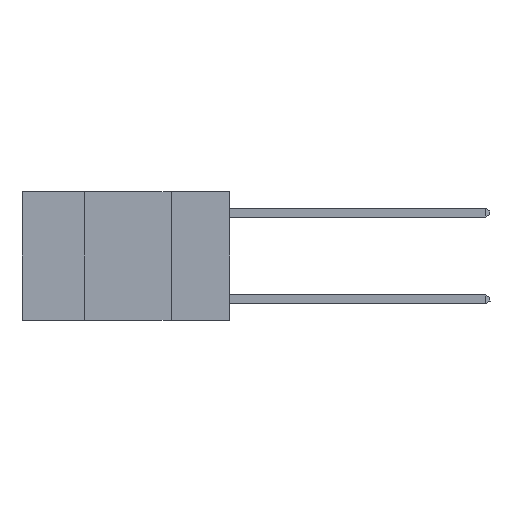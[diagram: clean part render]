
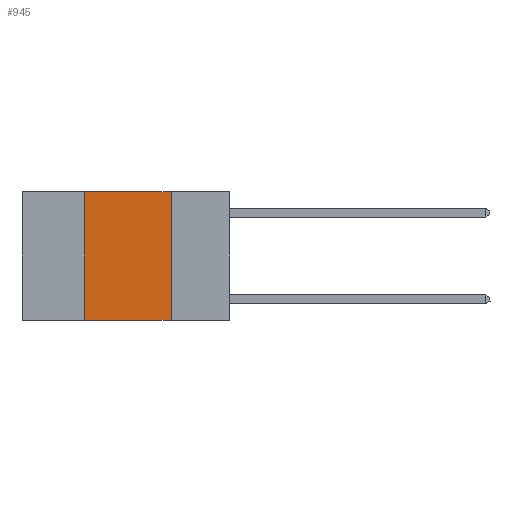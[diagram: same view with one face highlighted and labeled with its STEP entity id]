
A CAD part, left-side view. The second image highlights one B-rep face of the part: STEP entity #945.
In plain terms, the highlighted planar face has unit normal (-1, 0, 0).
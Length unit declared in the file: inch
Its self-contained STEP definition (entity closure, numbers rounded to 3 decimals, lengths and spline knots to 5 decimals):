
#25 = VECTOR ( 'NONE', #1550, 39.37008 ) ;
#100 = EDGE_CURVE ( 'NONE', #499, #8716, #5270, .T. ) ;
#407 = DIRECTION ( 'NONE',  ( 0., -1., 0. ) ) ;
#499 = VERTEX_POINT ( 'NONE', #9473 ) ;
#731 = CARTESIAN_POINT ( 'NONE',  ( 0., 0.17, 0. ) ) ;
#945 = ADVANCED_FACE ( 'NONE', ( #7794 ), #3126, .F. ) ;
#1162 = EDGE_CURVE ( 'NONE', #499, #2624, #2180, .T. ) ;
#1550 = DIRECTION ( 'NONE',  ( 0., 0., -1. ) ) ;
#1669 = VECTOR ( 'NONE', #8028, 39.37008 ) ;
#2180 = LINE ( 'NONE', #4954, #1669 ) ;
#2624 = VERTEX_POINT ( 'NONE', #5604 ) ;
#2625 = LINE ( 'NONE', #9827, #6765 ) ;
#2983 = CARTESIAN_POINT ( 'NONE',  ( 0., 0.17, -0.37 ) ) ;
#3094 = VERTEX_POINT ( 'NONE', #731 ) ;
#3126 = PLANE ( 'NONE',  #3746 ) ;
#3746 = AXIS2_PLACEMENT_3D ( 'NONE', #9336, #4681, #10117 ) ;
#4392 = DIRECTION ( 'NONE',  ( 0., -1., 0. ) ) ;
#4474 = EDGE_CURVE ( 'NONE', #3094, #8716, #6290, .T. ) ;
#4681 = DIRECTION ( 'NONE',  ( 1., 0., 0. ) ) ;
#4954 = CARTESIAN_POINT ( 'NONE',  ( 0., 0.42, 0. ) ) ;
#5026 = ORIENTED_EDGE ( 'NONE', *, *, #4474, .F. ) ;
#5064 = ORIENTED_EDGE ( 'NONE', *, *, #100, .T. ) ;
#5115 = CARTESIAN_POINT ( 'NONE',  ( 0., 0.6, -0.37 ) ) ;
#5270 = LINE ( 'NONE', #5115, #7076 ) ;
#5604 = CARTESIAN_POINT ( 'NONE',  ( 0., 0.42, 0. ) ) ;
#5927 = EDGE_CURVE ( 'NONE', #2624, #3094, #2625, .T. ) ;
#6225 = ORIENTED_EDGE ( 'NONE', *, *, #1162, .F. ) ;
#6290 = LINE ( 'NONE', #7019, #25 ) ;
#6418 = EDGE_LOOP ( 'NONE', ( #5026, #7607, #6225, #5064 ) ) ;
#6765 = VECTOR ( 'NONE', #4392, 39.37008 ) ;
#7019 = CARTESIAN_POINT ( 'NONE',  ( 0., 0.17, 0. ) ) ;
#7076 = VECTOR ( 'NONE', #407, 39.37008 ) ;
#7607 = ORIENTED_EDGE ( 'NONE', *, *, #5927, .F. ) ;
#7794 = FACE_OUTER_BOUND ( 'NONE', #6418, .T. ) ;
#8028 = DIRECTION ( 'NONE',  ( 0., 0., 1. ) ) ;
#8716 = VERTEX_POINT ( 'NONE', #2983 ) ;
#9336 = CARTESIAN_POINT ( 'NONE',  ( 0., 0.6, 0. ) ) ;
#9473 = CARTESIAN_POINT ( 'NONE',  ( 0., 0.42, -0.37 ) ) ;
#9827 = CARTESIAN_POINT ( 'NONE',  ( 0., 0.6, 0. ) ) ;
#10117 = DIRECTION ( 'NONE',  ( 0., 0., -1. ) ) ;
